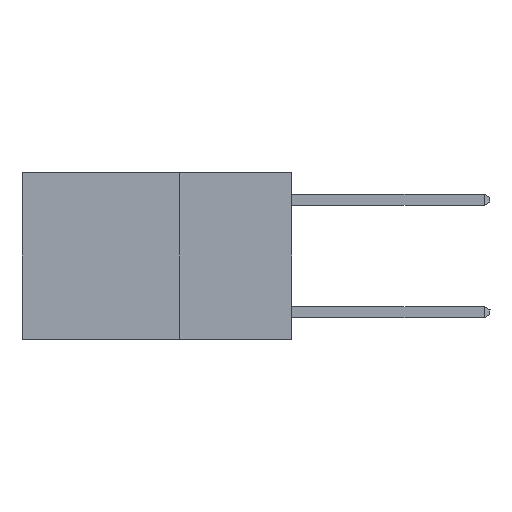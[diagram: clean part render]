
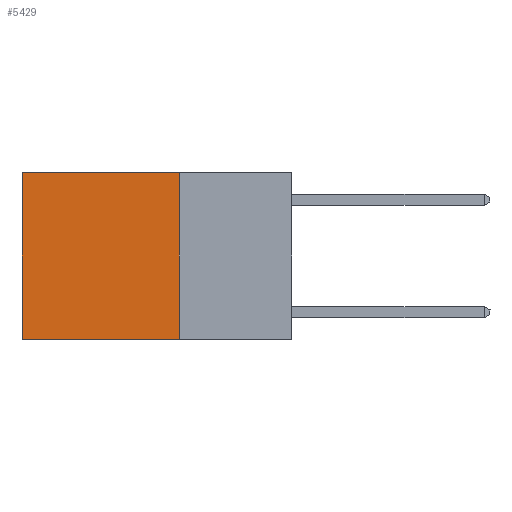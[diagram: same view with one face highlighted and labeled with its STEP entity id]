
A CAD part, left-side view. The second image highlights one B-rep face of the part: STEP entity #5429.
In plain terms, the highlighted planar face has unit normal (-1, 0, 0).
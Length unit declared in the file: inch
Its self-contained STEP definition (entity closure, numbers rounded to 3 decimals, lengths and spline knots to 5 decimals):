
#97 = DIRECTION ( 'NONE',  ( 1., 0., 0. ) ) ;
#1332 = VERTEX_POINT ( 'NONE', #19855 ) ;
#1578 = VECTOR ( 'NONE', #4383, 39.37008 ) ;
#2587 = LINE ( 'NONE', #17952, #14835 ) ;
#3040 = CARTESIAN_POINT ( 'NONE',  ( 0.2625, 0.25, 0. ) ) ;
#3306 = EDGE_CURVE ( 'NONE', #1332, #16047, #16826, .T. ) ;
#3848 = DIRECTION ( 'NONE',  ( 0., 0., -1. ) ) ;
#4383 = DIRECTION ( 'NONE',  ( 0., 1., 0. ) ) ;
#4483 = ORIENTED_EDGE ( 'NONE', *, *, #5169, .T. ) ;
#5115 = VECTOR ( 'NONE', #6178, 39.37008 ) ;
#5169 = EDGE_CURVE ( 'NONE', #13470, #16047, #2587, .T. ) ;
#5429 = ADVANCED_FACE ( 'NONE', ( #14587 ), #6846, .F. ) ;
#5805 = CARTESIAN_POINT ( 'NONE',  ( 0.2625, 0.25, 0. ) ) ;
#5922 = CARTESIAN_POINT ( 'NONE',  ( 0.2625, 0.25, -0.37 ) ) ;
#6178 = DIRECTION ( 'NONE',  ( 0., 1., 0. ) ) ;
#6846 = PLANE ( 'NONE',  #8307 ) ;
#7293 = CARTESIAN_POINT ( 'NONE',  ( 0.2625, 0.25, 0. ) ) ;
#8307 = AXIS2_PLACEMENT_3D ( 'NONE', #8464, #97, #3848 ) ;
#8464 = CARTESIAN_POINT ( 'NONE',  ( 0.2625, 0.25, 0. ) ) ;
#8644 = DIRECTION ( 'NONE',  ( 0., 0., -1. ) ) ;
#9274 = ORIENTED_EDGE ( 'NONE', *, *, #16550, .T. ) ;
#11344 = CARTESIAN_POINT ( 'NONE',  ( 0.2625, 0.6, 0. ) ) ;
#13147 = ORIENTED_EDGE ( 'NONE', *, *, #3306, .F. ) ;
#13470 = VERTEX_POINT ( 'NONE', #11344 ) ;
#13830 = VERTEX_POINT ( 'NONE', #5805 ) ;
#14355 = LINE ( 'NONE', #3040, #5115 ) ;
#14587 = FACE_OUTER_BOUND ( 'NONE', #18749, .T. ) ;
#14835 = VECTOR ( 'NONE', #8644, 39.37008 ) ;
#15461 = DIRECTION ( 'NONE',  ( 0., 0., -1. ) ) ;
#15556 = ORIENTED_EDGE ( 'NONE', *, *, #18967, .F. ) ;
#16047 = VERTEX_POINT ( 'NONE', #19109 ) ;
#16550 = EDGE_CURVE ( 'NONE', #13830, #13470, #14355, .T. ) ;
#16826 = LINE ( 'NONE', #5922, #1578 ) ;
#17952 = CARTESIAN_POINT ( 'NONE',  ( 0.2625, 0.6, 0. ) ) ;
#18202 = VECTOR ( 'NONE', #15461, 39.37008 ) ;
#18749 = EDGE_LOOP ( 'NONE', ( #4483, #13147, #15556, #9274 ) ) ;
#18967 = EDGE_CURVE ( 'NONE', #13830, #1332, #18974, .T. ) ;
#18974 = LINE ( 'NONE', #7293, #18202 ) ;
#19109 = CARTESIAN_POINT ( 'NONE',  ( 0.2625, 0.6, -0.37 ) ) ;
#19855 = CARTESIAN_POINT ( 'NONE',  ( 0.2625, 0.25, -0.37 ) ) ;
